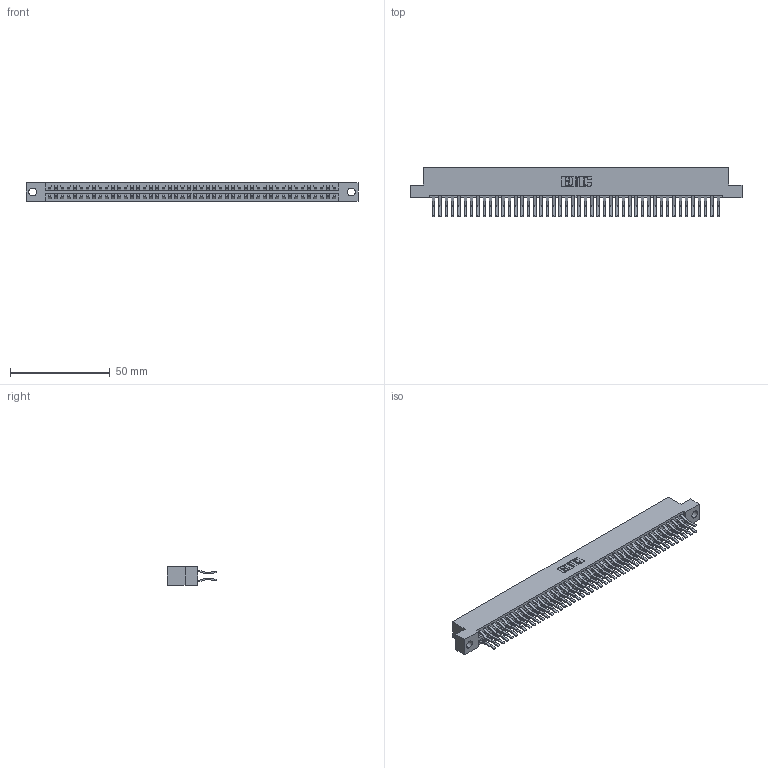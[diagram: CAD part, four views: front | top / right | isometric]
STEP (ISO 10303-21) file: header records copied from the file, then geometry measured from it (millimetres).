
FILE_DESCRIPTION (( 'STEP AP203' ), '1' );
FILE_NAME ('346-092-560-204.STEP', '2022-05-26T08:46:25', ( '' ), ( '' ), 'SwSTEP 2.0', 'SolidWorks 2020', '' );
FILE_SCHEMA (( 'CONFIG_CONTROL_DESIGN' ));
Length unit declared in the file: inch
Products named in the file (3): 346-092-560-204; 346 Part_Flush Mounting Lugs - 0.156 Dia-TH; 345-292-001_560 Tail
Assembly tree (93 placements, depth 2):
  346-092-560-204
    346 Part_Flush Mounting Lugs - 0.156 Dia-TH
    345-292-001_560 Tail  x92
Bounding box: 166.62 x 24.78 x 9.4 mm (x, y, z)
Volume: 16776.1 mm3; surface area: 24579.4 mm2
Topology: 93 solids, 93 shells, 5104 faces, 15177 edges, 9994 vertices
Faces by surface type: plane 3310, cylinder 1794
Entity records: 29989 total; most frequent: CARTESIAN_POINT 4942, ORIENTED_EDGE 4874, DIRECTION 4409, EDGE_CURVE 2437, VECTOR 2117, LINE 2117, VERTEX_POINT 1622, AXIS2_PLACEMENT_3D 1146
